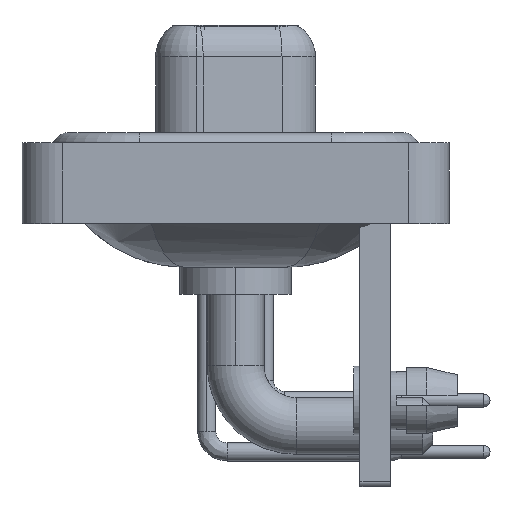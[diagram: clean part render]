
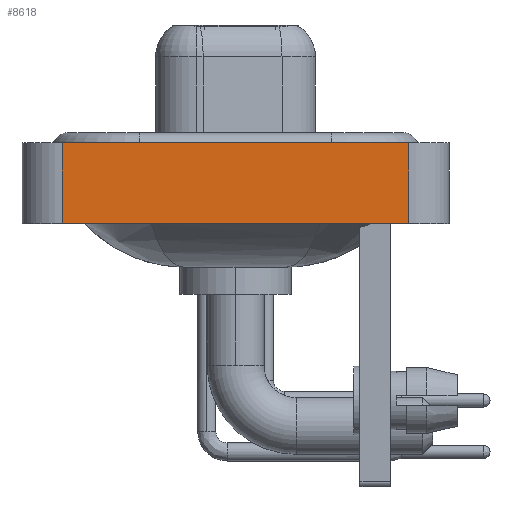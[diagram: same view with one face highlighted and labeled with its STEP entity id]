
A CAD part, left-side view. The second image highlights one B-rep face of the part: STEP entity #8618.
In plain terms, the highlighted planar face has unit normal (-1, 0, 0).
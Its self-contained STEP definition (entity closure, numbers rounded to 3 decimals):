
#2256 = ORIENTED_EDGE ( 'NONE', *, *, #14264, .F. ) ;
#2421 = LINE ( 'NONE', #5682, #16714 ) ;
#3044 = ORIENTED_EDGE ( 'NONE', *, *, #18952, .T. ) ;
#3365 = VECTOR ( 'NONE', #15084, 1000. ) ;
#3379 = DIRECTION ( 'NONE',  ( 0., 0., 1. ) ) ;
#5628 = DIRECTION ( 'NONE',  ( -1., 0., 0. ) ) ;
#5682 = CARTESIAN_POINT ( 'NONE',  ( -7.3, -8.55, 0.4 ) ) ;
#5757 = LINE ( 'NONE', #7956, #3365 ) ;
#6607 = VERTEX_POINT ( 'NONE', #13272 ) ;
#6731 = VECTOR ( 'NONE', #8275, 1000. ) ;
#6873 = VERTEX_POINT ( 'NONE', #12674 ) ;
#7138 = AXIS2_PLACEMENT_3D ( 'NONE', #21632, #5628, #12770 ) ;
#7471 = EDGE_CURVE ( 'NONE', #8445, #17124, #5757, .T. ) ;
#7956 = CARTESIAN_POINT ( 'NONE',  ( -7.3, -8.55, -3.6 ) ) ;
#8275 = DIRECTION ( 'NONE',  ( 0., 0., 1. ) ) ;
#8445 = VERTEX_POINT ( 'NONE', #17553 ) ;
#8618 = ADVANCED_FACE ( 'NONE', ( #18006 ), #14505, .T. ) ;
#9038 = EDGE_LOOP ( 'NONE', ( #3044, #10007, #2256, #14550 ) ) ;
#9778 = CARTESIAN_POINT ( 'NONE',  ( -7.3, -8.55, -3.6 ) ) ;
#10007 = ORIENTED_EDGE ( 'NONE', *, *, #16150, .F. ) ;
#12674 = CARTESIAN_POINT ( 'NONE',  ( -7.3, -8.55, 0.4 ) ) ;
#12770 = DIRECTION ( 'NONE',  ( 0., 0., 1. ) ) ;
#13083 = VECTOR ( 'NONE', #3379, 1000. ) ;
#13272 = CARTESIAN_POINT ( 'NONE',  ( -7.3, 8.55, 0.4 ) ) ;
#13291 = CARTESIAN_POINT ( 'NONE',  ( -7.3, -8.55, -3.6 ) ) ;
#14264 = EDGE_CURVE ( 'NONE', #8445, #6607, #17743, .T. ) ;
#14441 = DIRECTION ( 'NONE',  ( 0., -1., 0. ) ) ;
#14505 = PLANE ( 'NONE',  #7138 ) ;
#14550 = ORIENTED_EDGE ( 'NONE', *, *, #7471, .T. ) ;
#15084 = DIRECTION ( 'NONE',  ( 0., -1., 0. ) ) ;
#16150 = EDGE_CURVE ( 'NONE', #6607, #6873, #2421, .T. ) ;
#16714 = VECTOR ( 'NONE', #14441, 1000. ) ;
#17124 = VERTEX_POINT ( 'NONE', #13291 ) ;
#17553 = CARTESIAN_POINT ( 'NONE',  ( -7.3, 8.55, -3.6 ) ) ;
#17743 = LINE ( 'NONE', #19624, #13083 ) ;
#18006 = FACE_OUTER_BOUND ( 'NONE', #9038, .T. ) ;
#18787 = LINE ( 'NONE', #9778, #6731 ) ;
#18952 = EDGE_CURVE ( 'NONE', #17124, #6873, #18787, .T. ) ;
#19624 = CARTESIAN_POINT ( 'NONE',  ( -7.3, 8.55, -3.6 ) ) ;
#21632 = CARTESIAN_POINT ( 'NONE',  ( -7.3, -8.55, -3.6 ) ) ;
